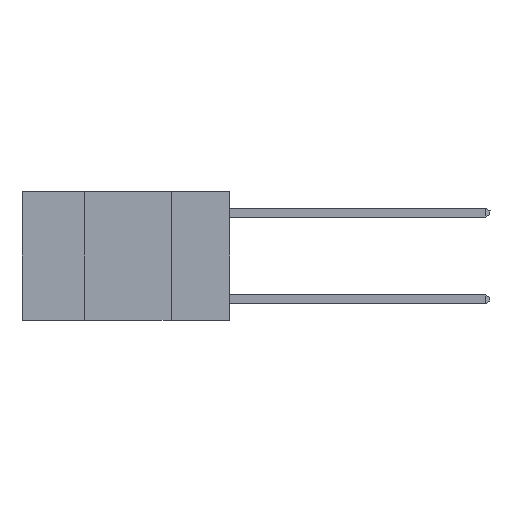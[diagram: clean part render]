
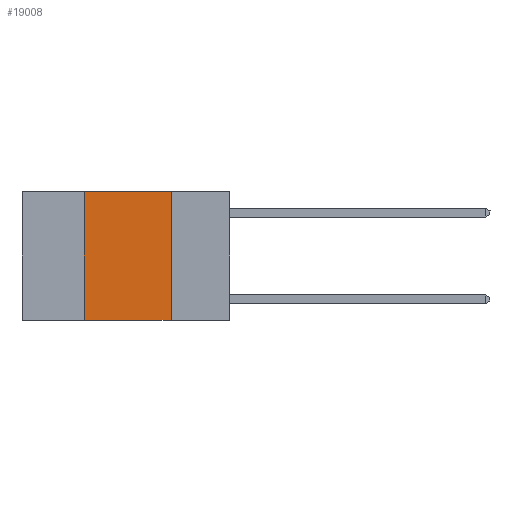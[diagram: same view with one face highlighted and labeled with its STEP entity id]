
A CAD part, left-side view. The second image highlights one B-rep face of the part: STEP entity #19008.
In plain terms, the highlighted planar face has unit normal (-1, 0, 0).
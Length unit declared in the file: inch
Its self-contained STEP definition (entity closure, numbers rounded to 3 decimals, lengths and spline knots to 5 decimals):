
#407 = DIRECTION ( 'NONE',  ( 0., -1., 0. ) ) ;
#862 = DIRECTION ( 'NONE',  ( 0., 0., -1. ) ) ;
#1117 = CARTESIAN_POINT ( 'NONE',  ( 0., 0.17, 0. ) ) ;
#1208 = VERTEX_POINT ( 'NONE', #18057 ) ;
#2521 = VERTEX_POINT ( 'NONE', #18480 ) ;
#2524 = ORIENTED_EDGE ( 'NONE', *, *, #8197, .F. ) ;
#2830 = ORIENTED_EDGE ( 'NONE', *, *, #6712, .F. ) ;
#5307 = DIRECTION ( 'NONE',  ( 1., 0., 0. ) ) ;
#5452 = EDGE_CURVE ( 'NONE', #2521, #1208, #12650, .T. ) ;
#6641 = CARTESIAN_POINT ( 'NONE',  ( 0., 0.42, 0. ) ) ;
#6712 = EDGE_CURVE ( 'NONE', #7228, #1208, #18387, .T. ) ;
#7228 = VERTEX_POINT ( 'NONE', #22256 ) ;
#7336 = VERTEX_POINT ( 'NONE', #20998 ) ;
#8197 = EDGE_CURVE ( 'NONE', #2521, #7336, #17527, .T. ) ;
#9126 = ORIENTED_EDGE ( 'NONE', *, *, #13844, .F. ) ;
#9588 = DIRECTION ( 'NONE',  ( 0., 0., -1. ) ) ;
#10681 = DIRECTION ( 'NONE',  ( 0., -1., 0. ) ) ;
#11291 = PLANE ( 'NONE',  #12265 ) ;
#12265 = AXIS2_PLACEMENT_3D ( 'NONE', #19682, #5307, #862 ) ;
#12300 = VECTOR ( 'NONE', #21845, 39.37008 ) ;
#12638 = VECTOR ( 'NONE', #10681, 39.37008 ) ;
#12650 = LINE ( 'NONE', #16693, #12638 ) ;
#13844 = EDGE_CURVE ( 'NONE', #7336, #7228, #26165, .T. ) ;
#16416 = ORIENTED_EDGE ( 'NONE', *, *, #5452, .T. ) ;
#16693 = CARTESIAN_POINT ( 'NONE',  ( 0., 0.6, -0.37 ) ) ;
#17098 = EDGE_LOOP ( 'NONE', ( #2830, #9126, #2524, #16416 ) ) ;
#17127 = CARTESIAN_POINT ( 'NONE',  ( 0., 0.6, 0. ) ) ;
#17527 = LINE ( 'NONE', #6641, #12300 ) ;
#18057 = CARTESIAN_POINT ( 'NONE',  ( 0., 0.17, -0.37 ) ) ;
#18387 = LINE ( 'NONE', #1117, #23416 ) ;
#18480 = CARTESIAN_POINT ( 'NONE',  ( 0., 0.42, -0.37 ) ) ;
#19008 = ADVANCED_FACE ( 'NONE', ( #22469 ), #11291, .F. ) ;
#19682 = CARTESIAN_POINT ( 'NONE',  ( 0., 0.6, 0. ) ) ;
#20998 = CARTESIAN_POINT ( 'NONE',  ( 0., 0.42, 0. ) ) ;
#21845 = DIRECTION ( 'NONE',  ( 0., 0., 1. ) ) ;
#22256 = CARTESIAN_POINT ( 'NONE',  ( 0., 0.17, 0. ) ) ;
#22469 = FACE_OUTER_BOUND ( 'NONE', #17098, .T. ) ;
#23416 = VECTOR ( 'NONE', #9588, 39.37008 ) ;
#26165 = LINE ( 'NONE', #17127, #26790 ) ;
#26790 = VECTOR ( 'NONE', #407, 39.37008 ) ;
